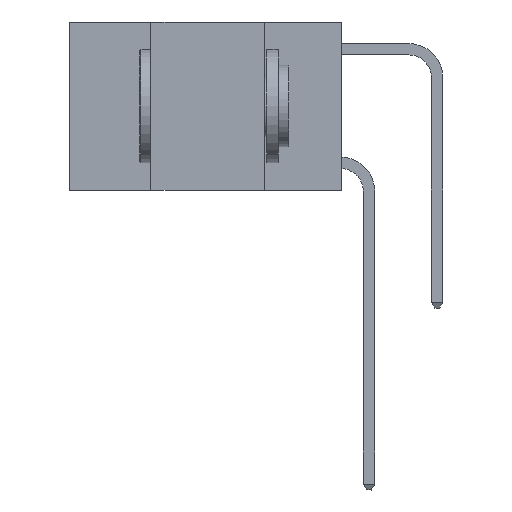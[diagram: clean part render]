
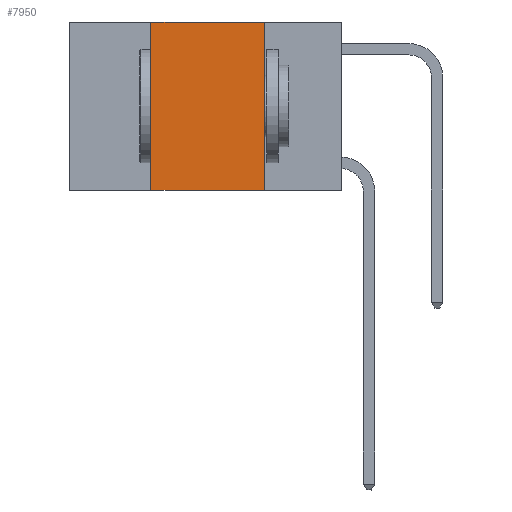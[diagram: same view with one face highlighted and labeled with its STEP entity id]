
A CAD part, left-side view. The second image highlights one B-rep face of the part: STEP entity #7950.
In plain terms, the highlighted planar face has unit normal (-1, 0, 0).
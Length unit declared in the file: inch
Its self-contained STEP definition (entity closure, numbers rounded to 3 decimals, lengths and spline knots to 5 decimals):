
#70 = VERTEX_POINT ( 'NONE', #1773 ) ;
#304 = DIRECTION ( 'NONE',  ( 0., 0., -1. ) ) ;
#1304 = VERTEX_POINT ( 'NONE', #2145 ) ;
#1657 = LINE ( 'NONE', #4678, #3954 ) ;
#1773 = CARTESIAN_POINT ( 'NONE',  ( 0., 0.17, -0.37 ) ) ;
#2145 = CARTESIAN_POINT ( 'NONE',  ( 0., 0.17, 0. ) ) ;
#2507 = VERTEX_POINT ( 'NONE', #11450 ) ;
#3158 = ORIENTED_EDGE ( 'NONE', *, *, #5063, .F. ) ;
#3489 = EDGE_CURVE ( 'NONE', #2507, #70, #4445, .T. ) ;
#3954 = VECTOR ( 'NONE', #9498, 39.37008 ) ;
#4188 = CARTESIAN_POINT ( 'NONE',  ( 0., 0.6, 0. ) ) ;
#4445 = LINE ( 'NONE', #10411, #11764 ) ;
#4678 = CARTESIAN_POINT ( 'NONE',  ( 0., 0.42, 0. ) ) ;
#5029 = EDGE_CURVE ( 'NONE', #1304, #70, #9035, .T. ) ;
#5063 = EDGE_CURVE ( 'NONE', #10085, #1304, #11816, .T. ) ;
#6049 = DIRECTION ( 'NONE',  ( 1., 0., 0. ) ) ;
#6121 = VECTOR ( 'NONE', #8853, 39.37008 ) ;
#6912 = EDGE_LOOP ( 'NONE', ( #12268, #3158, #8169, #9756 ) ) ;
#6995 = PLANE ( 'NONE',  #10705 ) ;
#7552 = CARTESIAN_POINT ( 'NONE',  ( 0., 0.6, 0. ) ) ;
#7950 = ADVANCED_FACE ( 'NONE', ( #11012 ), #6995, .F. ) ;
#8169 = ORIENTED_EDGE ( 'NONE', *, *, #11610, .F. ) ;
#8776 = CARTESIAN_POINT ( 'NONE',  ( 0., 0.42, 0. ) ) ;
#8853 = DIRECTION ( 'NONE',  ( 0., -1., 0. ) ) ;
#9019 = DIRECTION ( 'NONE',  ( 0., 0., -1. ) ) ;
#9035 = LINE ( 'NONE', #9432, #11532 ) ;
#9432 = CARTESIAN_POINT ( 'NONE',  ( 0., 0.17, 0. ) ) ;
#9498 = DIRECTION ( 'NONE',  ( 0., 0., 1. ) ) ;
#9756 = ORIENTED_EDGE ( 'NONE', *, *, #3489, .T. ) ;
#10085 = VERTEX_POINT ( 'NONE', #8776 ) ;
#10411 = CARTESIAN_POINT ( 'NONE',  ( 0., 0.6, -0.37 ) ) ;
#10705 = AXIS2_PLACEMENT_3D ( 'NONE', #4188, #6049, #304 ) ;
#10957 = DIRECTION ( 'NONE',  ( 0., -1., 0. ) ) ;
#11012 = FACE_OUTER_BOUND ( 'NONE', #6912, .T. ) ;
#11450 = CARTESIAN_POINT ( 'NONE',  ( 0., 0.42, -0.37 ) ) ;
#11532 = VECTOR ( 'NONE', #9019, 39.37008 ) ;
#11610 = EDGE_CURVE ( 'NONE', #2507, #10085, #1657, .T. ) ;
#11764 = VECTOR ( 'NONE', #10957, 39.37008 ) ;
#11816 = LINE ( 'NONE', #7552, #6121 ) ;
#12268 = ORIENTED_EDGE ( 'NONE', *, *, #5029, .F. ) ;
